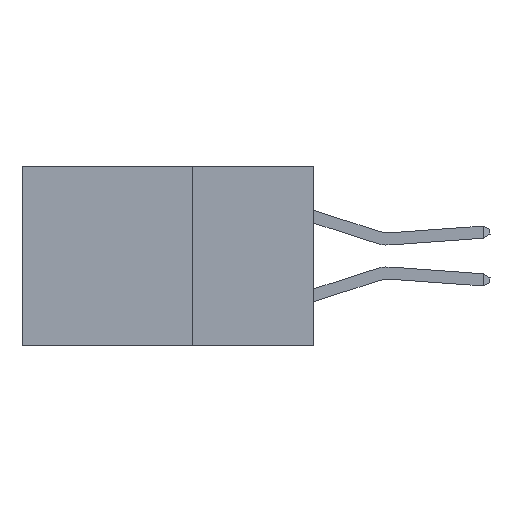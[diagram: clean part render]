
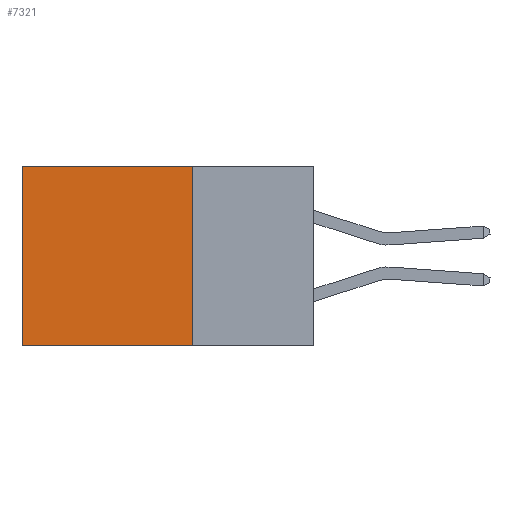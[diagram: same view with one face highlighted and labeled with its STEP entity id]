
A CAD part, left-side view. The second image highlights one B-rep face of the part: STEP entity #7321.
In plain terms, the highlighted planar face has unit normal (-1, 0, 0).
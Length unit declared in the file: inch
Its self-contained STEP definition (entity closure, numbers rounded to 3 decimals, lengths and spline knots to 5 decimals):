
#263 = CARTESIAN_POINT ( 'NONE',  ( 0.2875, 0.25, 0. ) ) ;
#361 = ORIENTED_EDGE ( 'NONE', *, *, #3656, .T. ) ;
#403 = CARTESIAN_POINT ( 'NONE',  ( 0.2875, 0.25, 0. ) ) ;
#555 = CARTESIAN_POINT ( 'NONE',  ( 0.2875, 0.6, 0. ) ) ;
#589 = DIRECTION ( 'NONE',  ( 0., 0., -1. ) ) ;
#646 = CARTESIAN_POINT ( 'NONE',  ( 0.2875, 0.6, -0.37 ) ) ;
#1181 = VECTOR ( 'NONE', #8245, 39.37008 ) ;
#1386 = ORIENTED_EDGE ( 'NONE', *, *, #13726, .F. ) ;
#1487 = VERTEX_POINT ( 'NONE', #17042 ) ;
#1494 = VERTEX_POINT ( 'NONE', #16047 ) ;
#1795 = DIRECTION ( 'NONE',  ( 0., 0., -1. ) ) ;
#2317 = ORIENTED_EDGE ( 'NONE', *, *, #15644, .T. ) ;
#3107 = VERTEX_POINT ( 'NONE', #555 ) ;
#3326 = DIRECTION ( 'NONE',  ( 0., 1., 0. ) ) ;
#3656 = EDGE_CURVE ( 'NONE', #3107, #6763, #16257, .T. ) ;
#4073 = LINE ( 'NONE', #403, #9958 ) ;
#6195 = DIRECTION ( 'NONE',  ( 0., 0., -1. ) ) ;
#6484 = AXIS2_PLACEMENT_3D ( 'NONE', #263, #9949, #1795 ) ;
#6763 = VERTEX_POINT ( 'NONE', #646 ) ;
#7136 = VECTOR ( 'NONE', #589, 39.37008 ) ;
#7321 = ADVANCED_FACE ( 'NONE', ( #10393 ), #12511, .F. ) ;
#7858 = ORIENTED_EDGE ( 'NONE', *, *, #12769, .F. ) ;
#8245 = DIRECTION ( 'NONE',  ( 0., 1., 0. ) ) ;
#9031 = VECTOR ( 'NONE', #6195, 39.37008 ) ;
#9949 = DIRECTION ( 'NONE',  ( 1., 0., 0. ) ) ;
#9958 = VECTOR ( 'NONE', #3326, 39.37008 ) ;
#10393 = FACE_OUTER_BOUND ( 'NONE', #11760, .T. ) ;
#11551 = CARTESIAN_POINT ( 'NONE',  ( 0.2875, 0.25, 0. ) ) ;
#11760 = EDGE_LOOP ( 'NONE', ( #361, #1386, #7858, #2317 ) ) ;
#12024 = LINE ( 'NONE', #12121, #1181 ) ;
#12121 = CARTESIAN_POINT ( 'NONE',  ( 0.2875, 0.25, -0.37 ) ) ;
#12511 = PLANE ( 'NONE',  #6484 ) ;
#12769 = EDGE_CURVE ( 'NONE', #1487, #1494, #17021, .T. ) ;
#13726 = EDGE_CURVE ( 'NONE', #1494, #6763, #12024, .T. ) ;
#15250 = CARTESIAN_POINT ( 'NONE',  ( 0.2875, 0.6, 0. ) ) ;
#15644 = EDGE_CURVE ( 'NONE', #1487, #3107, #4073, .T. ) ;
#16047 = CARTESIAN_POINT ( 'NONE',  ( 0.2875, 0.25, -0.37 ) ) ;
#16257 = LINE ( 'NONE', #15250, #9031 ) ;
#17021 = LINE ( 'NONE', #11551, #7136 ) ;
#17042 = CARTESIAN_POINT ( 'NONE',  ( 0.2875, 0.25, 0. ) ) ;
